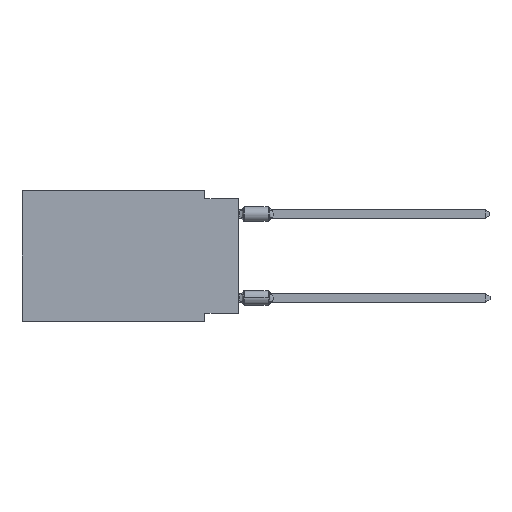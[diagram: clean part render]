
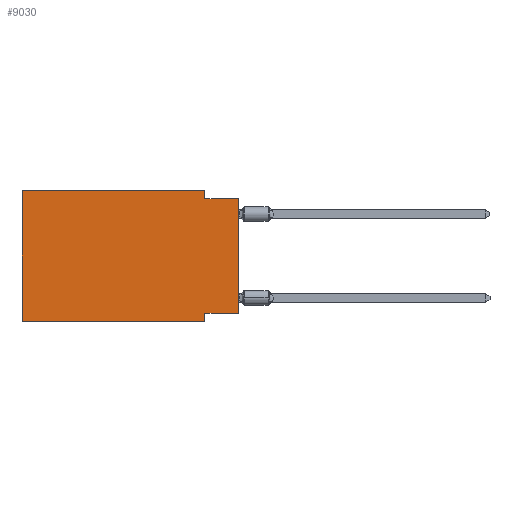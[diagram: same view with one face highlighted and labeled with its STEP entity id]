
A CAD part, left-side view. The second image highlights one B-rep face of the part: STEP entity #9030.
In plain terms, the highlighted planar face has unit normal (-1, 0, 0).
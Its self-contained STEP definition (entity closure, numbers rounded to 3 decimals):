
#385 = VERTEX_POINT ( 'NONE', #16575 ) ;
#448 = ORIENTED_EDGE ( 'NONE', *, *, #7396, .F. ) ;
#726 = CARTESIAN_POINT ( 'NONE',  ( 0., 16.383, -9.906 ) ) ;
#826 = CARTESIAN_POINT ( 'NONE',  ( 0., 0., -9.271 ) ) ;
#1309 = EDGE_CURVE ( 'NONE', #4933, #8884, #17027, .T. ) ;
#1318 = DIRECTION ( 'NONE',  ( 0., -1., 0. ) ) ;
#1765 = EDGE_CURVE ( 'NONE', #385, #14768, #5358, .T. ) ;
#2039 = FACE_OUTER_BOUND ( 'NONE', #13935, .T. ) ;
#2398 = ORIENTED_EDGE ( 'NONE', *, *, #11325, .T. ) ;
#3071 = DIRECTION ( 'NONE',  ( 0., -1., 0. ) ) ;
#3284 = CARTESIAN_POINT ( 'NONE',  ( 0., 2.54, 0. ) ) ;
#3810 = DIRECTION ( 'NONE',  ( 0., 0., 1. ) ) ;
#4933 = VERTEX_POINT ( 'NONE', #16860 ) ;
#4963 = CARTESIAN_POINT ( 'NONE',  ( 0., 16.383, 0. ) ) ;
#5164 = CARTESIAN_POINT ( 'NONE',  ( 0., 2.54, -9.906 ) ) ;
#5236 = VERTEX_POINT ( 'NONE', #11366 ) ;
#5358 = LINE ( 'NONE', #10834, #10290 ) ;
#5689 = VECTOR ( 'NONE', #10198, 1000. ) ;
#5854 = ORIENTED_EDGE ( 'NONE', *, *, #16086, .F. ) ;
#6280 = ORIENTED_EDGE ( 'NONE', *, *, #9424, .T. ) ;
#7098 = PLANE ( 'NONE',  #14821 ) ;
#7099 = VECTOR ( 'NONE', #1318, 1000. ) ;
#7267 = DIRECTION ( 'NONE',  ( 0., 0., 1. ) ) ;
#7396 = EDGE_CURVE ( 'NONE', #8884, #385, #15179, .T. ) ;
#7488 = EDGE_CURVE ( 'NONE', #15619, #4933, #16642, .T. ) ;
#7746 = CARTESIAN_POINT ( 'NONE',  ( 0., 2.54, 0. ) ) ;
#8079 = VERTEX_POINT ( 'NONE', #826 ) ;
#8681 = LINE ( 'NONE', #10069, #12338 ) ;
#8884 = VERTEX_POINT ( 'NONE', #7746 ) ;
#8892 = LINE ( 'NONE', #5164, #5689 ) ;
#9030 = ADVANCED_FACE ( 'NONE', ( #2039 ), #7098, .F. ) ;
#9394 = VECTOR ( 'NONE', #7267, 1000. ) ;
#9424 = EDGE_CURVE ( 'NONE', #15619, #15946, #12618, .T. ) ;
#9910 = ORIENTED_EDGE ( 'NONE', *, *, #1765, .F. ) ;
#10069 = CARTESIAN_POINT ( 'NONE',  ( 0., 0., -9.271 ) ) ;
#10070 = EDGE_CURVE ( 'NONE', #8079, #5236, #8681, .T. ) ;
#10198 = DIRECTION ( 'NONE',  ( 0., 0., -1. ) ) ;
#10290 = VECTOR ( 'NONE', #14747, 1000. ) ;
#10399 = LINE ( 'NONE', #15709, #11549 ) ;
#10447 = ORIENTED_EDGE ( 'NONE', *, *, #10070, .F. ) ;
#10834 = CARTESIAN_POINT ( 'NONE',  ( 0., 0., -0.635 ) ) ;
#11325 = EDGE_CURVE ( 'NONE', #8079, #14768, #10399, .T. ) ;
#11366 = CARTESIAN_POINT ( 'NONE',  ( 0., 2.54, -9.271 ) ) ;
#11549 = VECTOR ( 'NONE', #3810, 1000. ) ;
#11901 = VECTOR ( 'NONE', #13798, 1000. ) ;
#12338 = VECTOR ( 'NONE', #13983, 1000. ) ;
#12479 = CARTESIAN_POINT ( 'NONE',  ( 0., 16.383, 0. ) ) ;
#12538 = DIRECTION ( 'NONE',  ( 1., 0., 0. ) ) ;
#12618 = LINE ( 'NONE', #726, #14276 ) ;
#13055 = ORIENTED_EDGE ( 'NONE', *, *, #7488, .F. ) ;
#13798 = DIRECTION ( 'NONE',  ( 0., 0., -1. ) ) ;
#13824 = ORIENTED_EDGE ( 'NONE', *, *, #1309, .F. ) ;
#13935 = EDGE_LOOP ( 'NONE', ( #2398, #9910, #448, #13824, #13055, #6280, #5854, #10447 ) ) ;
#13983 = DIRECTION ( 'NONE',  ( 0., 1., 0. ) ) ;
#14276 = VECTOR ( 'NONE', #3071, 1000. ) ;
#14453 = CARTESIAN_POINT ( 'NONE',  ( 0., 0., -0.635 ) ) ;
#14747 = DIRECTION ( 'NONE',  ( 0., -1., 0. ) ) ;
#14768 = VERTEX_POINT ( 'NONE', #14453 ) ;
#14821 = AXIS2_PLACEMENT_3D ( 'NONE', #16546, #12538, #15162 ) ;
#15162 = DIRECTION ( 'NONE',  ( 0., 0., -1. ) ) ;
#15179 = LINE ( 'NONE', #3284, #11901 ) ;
#15310 = CARTESIAN_POINT ( 'NONE',  ( 0., 2.54, -9.906 ) ) ;
#15619 = VERTEX_POINT ( 'NONE', #16820 ) ;
#15709 = CARTESIAN_POINT ( 'NONE',  ( 0., 0., 0. ) ) ;
#15946 = VERTEX_POINT ( 'NONE', #15310 ) ;
#16086 = EDGE_CURVE ( 'NONE', #5236, #15946, #8892, .T. ) ;
#16546 = CARTESIAN_POINT ( 'NONE',  ( 0., 16.383, 0. ) ) ;
#16575 = CARTESIAN_POINT ( 'NONE',  ( 0., 2.54, -0.635 ) ) ;
#16642 = LINE ( 'NONE', #12479, #9394 ) ;
#16820 = CARTESIAN_POINT ( 'NONE',  ( 0., 16.383, -9.906 ) ) ;
#16860 = CARTESIAN_POINT ( 'NONE',  ( 0., 16.383, 0. ) ) ;
#17027 = LINE ( 'NONE', #4963, #7099 ) ;
